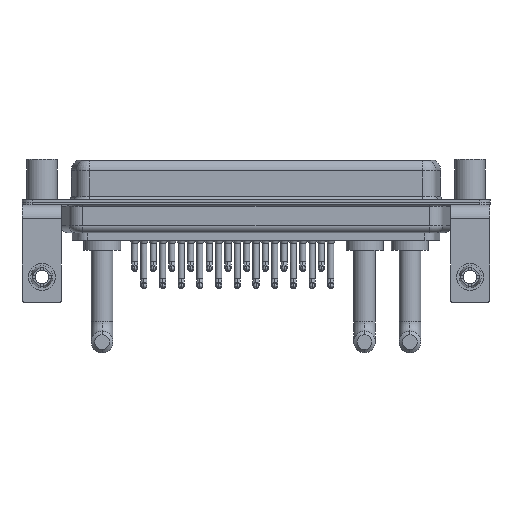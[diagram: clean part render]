
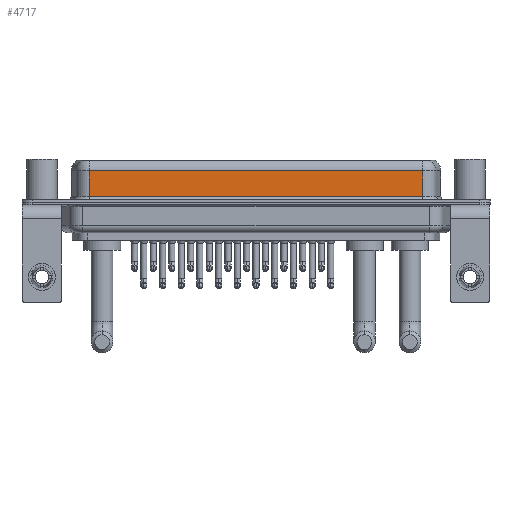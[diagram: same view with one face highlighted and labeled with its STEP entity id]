
A CAD part, front view. The second image highlights one B-rep face of the part: STEP entity #4717.
In plain terms, the highlighted planar face has unit normal (0, -1, 0).
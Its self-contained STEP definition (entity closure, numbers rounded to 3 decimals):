
#334 = ORIENTED_EDGE ( 'NONE', *, *, #15738, .T. ) ;
#2233 = AXIS2_PLACEMENT_3D ( 'NONE', #24919, #24788, #3345 ) ;
#2774 = ORIENTED_EDGE ( 'NONE', *, *, #16505, .T. ) ;
#3345 = DIRECTION ( 'NONE',  ( 0., 0., 1. ) ) ;
#3607 = VERTEX_POINT ( 'NONE', #6773 ) ;
#3738 = ORIENTED_EDGE ( 'NONE', *, *, #16581, .F. ) ;
#4717 = ADVANCED_FACE ( 'NONE', ( #22295 ), #11931, .F. ) ;
#5982 = DIRECTION ( 'NONE',  ( -1., 0., 0. ) ) ;
#6773 = CARTESIAN_POINT ( 'NONE',  ( 7.038, -3.95, 0.9 ) ) ;
#7357 = DIRECTION ( 'NONE',  ( 1., 0., 0. ) ) ;
#7446 = EDGE_LOOP ( 'NONE', ( #3738, #17763, #2774, #334 ) ) ;
#7908 = CARTESIAN_POINT ( 'NONE',  ( 56.462, -3.95, 0.9 ) ) ;
#8165 = VERTEX_POINT ( 'NONE', #7908 ) ;
#8738 = CARTESIAN_POINT ( 'NONE',  ( 56.462, -3.95, 4.65 ) ) ;
#9456 = CARTESIAN_POINT ( 'NONE',  ( 56.462, -3.95, 0.9 ) ) ;
#10514 = CARTESIAN_POINT ( 'NONE',  ( 7.038, -3.95, 6.4 ) ) ;
#10790 = DIRECTION ( 'NONE',  ( 0., 0., -1. ) ) ;
#11049 = VECTOR ( 'NONE', #7357, 1000. ) ;
#11206 = VERTEX_POINT ( 'NONE', #8738 ) ;
#11931 = PLANE ( 'NONE',  #2233 ) ;
#12392 = EDGE_CURVE ( 'NONE', #11206, #23044, #27015, .T. ) ;
#14651 = CARTESIAN_POINT ( 'NONE',  ( 56.462, -3.95, 6.4 ) ) ;
#15738 = EDGE_CURVE ( 'NONE', #3607, #8165, #21900, .T. ) ;
#15796 = VECTOR ( 'NONE', #5982, 1000. ) ;
#16505 = EDGE_CURVE ( 'NONE', #23044, #3607, #19466, .T. ) ;
#16581 = EDGE_CURVE ( 'NONE', #11206, #8165, #25433, .T. ) ;
#17763 = ORIENTED_EDGE ( 'NONE', *, *, #12392, .T. ) ;
#19466 = LINE ( 'NONE', #10514, #22517 ) ;
#21900 = LINE ( 'NONE', #9456, #11049 ) ;
#22295 = FACE_OUTER_BOUND ( 'NONE', #7446, .T. ) ;
#22517 = VECTOR ( 'NONE', #23228, 1000. ) ;
#23002 = CARTESIAN_POINT ( 'NONE',  ( 56.462, -3.95, 4.65 ) ) ;
#23044 = VERTEX_POINT ( 'NONE', #25149 ) ;
#23228 = DIRECTION ( 'NONE',  ( 0., 0., -1. ) ) ;
#24788 = DIRECTION ( 'NONE',  ( 0., 1., 0. ) ) ;
#24919 = CARTESIAN_POINT ( 'NONE',  ( 56.462, -3.95, 6.4 ) ) ;
#25149 = CARTESIAN_POINT ( 'NONE',  ( 7.038, -3.95, 4.65 ) ) ;
#25433 = LINE ( 'NONE', #14651, #26088 ) ;
#26088 = VECTOR ( 'NONE', #10790, 1000. ) ;
#27015 = LINE ( 'NONE', #23002, #15796 ) ;
